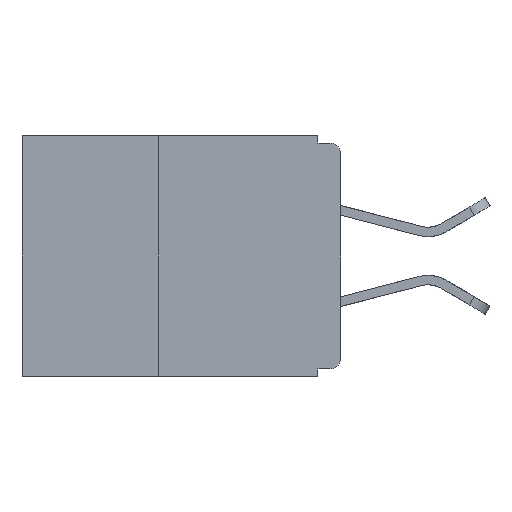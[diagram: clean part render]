
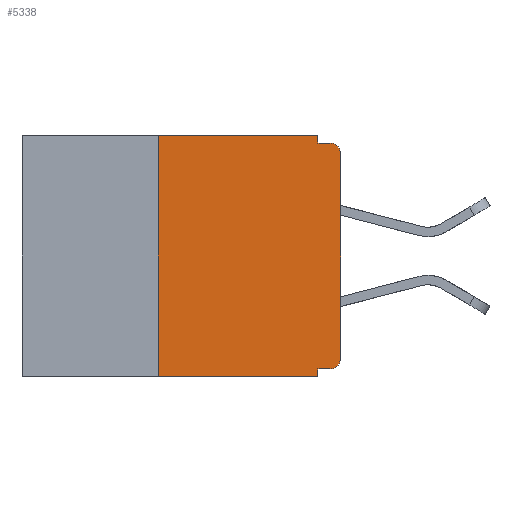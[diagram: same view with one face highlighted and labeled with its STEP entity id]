
A CAD part, left-side view. The second image highlights one B-rep face of the part: STEP entity #5338.
In plain terms, the highlighted planar face has unit normal (-1, 0, 0).
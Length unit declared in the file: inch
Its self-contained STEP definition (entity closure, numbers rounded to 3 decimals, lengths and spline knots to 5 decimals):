
#196 = VERTEX_POINT ( 'NONE', #17558 ) ;
#339 = VECTOR ( 'NONE', #9241, 39.37008 ) ;
#547 = VERTEX_POINT ( 'NONE', #24263 ) ;
#1603 = LINE ( 'NONE', #8749, #11624 ) ;
#1702 = EDGE_CURVE ( 'NONE', #196, #2056, #15099, .T. ) ;
#1730 = CARTESIAN_POINT ( 'NONE',  ( 0., 0.25, 0. ) ) ;
#2012 = CARTESIAN_POINT ( 'NONE',  ( 0., 0.25, -0.33 ) ) ;
#2056 = VERTEX_POINT ( 'NONE', #15801 ) ;
#2233 = LINE ( 'NONE', #6199, #12249 ) ;
#2402 = CIRCLE ( 'NONE', #25564, 0.015 ) ;
#2749 = ORIENTED_EDGE ( 'NONE', *, *, #4209, .T. ) ;
#2896 = CARTESIAN_POINT ( 'NONE',  ( 0., 0., -0.32 ) ) ;
#3173 = VERTEX_POINT ( 'NONE', #2012 ) ;
#3398 = LINE ( 'NONE', #2896, #12779 ) ;
#3401 = CARTESIAN_POINT ( 'NONE',  ( 0., 0.031, -0.32 ) ) ;
#3405 = ORIENTED_EDGE ( 'NONE', *, *, #19158, .F. ) ;
#4090 = EDGE_CURVE ( 'NONE', #4174, #18874, #1603, .T. ) ;
#4174 = VERTEX_POINT ( 'NONE', #6416 ) ;
#4209 = EDGE_CURVE ( 'NONE', #24738, #4174, #14375, .T. ) ;
#4511 = CARTESIAN_POINT ( 'NONE',  ( 0., 0.437, 0. ) ) ;
#4970 = ORIENTED_EDGE ( 'NONE', *, *, #14299, .T. ) ;
#4974 = VERTEX_POINT ( 'NONE', #3401 ) ;
#5245 = DIRECTION ( 'NONE',  ( 0., 0., -1. ) ) ;
#5330 = DIRECTION ( 'NONE',  ( -1., 0., 0. ) ) ;
#5338 = ADVANCED_FACE ( 'NONE', ( #14022 ), #20256, .F. ) ;
#5351 = DIRECTION ( 'NONE',  ( -1., 0., 0. ) ) ;
#5498 = CARTESIAN_POINT ( 'NONE',  ( 0., 0.015, -0.305 ) ) ;
#6107 = CARTESIAN_POINT ( 'NONE',  ( 0., 0.437, -0.33 ) ) ;
#6199 = CARTESIAN_POINT ( 'NONE',  ( 0., 0.031, -0.33 ) ) ;
#6416 = CARTESIAN_POINT ( 'NONE',  ( 0., 0., -0.305 ) ) ;
#6510 = DIRECTION ( 'NONE',  ( 1., 0., 0. ) ) ;
#6630 = AXIS2_PLACEMENT_3D ( 'NONE', #5498, #5330, #5245 ) ;
#7060 = DIRECTION ( 'NONE',  ( 0., 0., -1. ) ) ;
#7570 = LINE ( 'NONE', #6107, #25068 ) ;
#8061 = DIRECTION ( 'NONE',  ( 0., -1., 0. ) ) ;
#8165 = DIRECTION ( 'NONE',  ( 0., 0., 1. ) ) ;
#8234 = DIRECTION ( 'NONE',  ( 0., 0., -1. ) ) ;
#8249 = VECTOR ( 'NONE', #13335, 39.37008 ) ;
#8393 = ORIENTED_EDGE ( 'NONE', *, *, #1702, .F. ) ;
#8413 = ORIENTED_EDGE ( 'NONE', *, *, #14343, .F. ) ;
#8749 = CARTESIAN_POINT ( 'NONE',  ( 0., 0., 0. ) ) ;
#8942 = DIRECTION ( 'NONE',  ( 0., 1., 0. ) ) ;
#9241 = DIRECTION ( 'NONE',  ( 0., 0., 1. ) ) ;
#11624 = VECTOR ( 'NONE', #8165, 39.37008 ) ;
#12249 = VECTOR ( 'NONE', #8234, 39.37008 ) ;
#12487 = ORIENTED_EDGE ( 'NONE', *, *, #13399, .F. ) ;
#12779 = VECTOR ( 'NONE', #8942, 39.37008 ) ;
#12788 = ORIENTED_EDGE ( 'NONE', *, *, #24495, .T. ) ;
#13335 = DIRECTION ( 'NONE',  ( 0., -1., 0. ) ) ;
#13399 = EDGE_CURVE ( 'NONE', #16351, #547, #24535, .T. ) ;
#13924 = EDGE_LOOP ( 'NONE', ( #23977, #12788, #8393, #23773, #12487, #3405, #4970, #8413, #24376, #2749 ) ) ;
#14022 = FACE_OUTER_BOUND ( 'NONE', #13924, .T. ) ;
#14299 = EDGE_CURVE ( 'NONE', #3173, #17134, #7570, .T. ) ;
#14343 = EDGE_CURVE ( 'NONE', #4974, #17134, #2233, .T. ) ;
#14375 = CIRCLE ( 'NONE', #6630, 0.015 ) ;
#15099 = LINE ( 'NONE', #20082, #24827 ) ;
#15801 = CARTESIAN_POINT ( 'NONE',  ( 0., 0.015, -0.01 ) ) ;
#16240 = LINE ( 'NONE', #19032, #339 ) ;
#16351 = VERTEX_POINT ( 'NONE', #1730 ) ;
#16934 = CARTESIAN_POINT ( 'NONE',  ( 0., 0.031, 0. ) ) ;
#17134 = VERTEX_POINT ( 'NONE', #21874 ) ;
#17212 = CARTESIAN_POINT ( 'NONE',  ( 0., 0.015, -0.025 ) ) ;
#17558 = CARTESIAN_POINT ( 'NONE',  ( 0., 0.031, -0.01 ) ) ;
#18874 = VERTEX_POINT ( 'NONE', #19456 ) ;
#19032 = CARTESIAN_POINT ( 'NONE',  ( 0., 0.25, -0.33 ) ) ;
#19158 = EDGE_CURVE ( 'NONE', #3173, #16351, #16240, .T. ) ;
#19178 = DIRECTION ( 'NONE',  ( 0., 0., -1. ) ) ;
#19456 = CARTESIAN_POINT ( 'NONE',  ( 0., 0., -0.025 ) ) ;
#20082 = CARTESIAN_POINT ( 'NONE',  ( 0., 0., -0.01 ) ) ;
#20228 = DIRECTION ( 'NONE',  ( 0., -1., 0. ) ) ;
#20256 = PLANE ( 'NONE',  #21041 ) ;
#20338 = DIRECTION ( 'NONE',  ( 0., 0., -1. ) ) ;
#21041 = AXIS2_PLACEMENT_3D ( 'NONE', #4511, #6510, #20338 ) ;
#21070 = LINE ( 'NONE', #16934, #25570 ) ;
#21547 = EDGE_CURVE ( 'NONE', #24738, #4974, #3398, .T. ) ;
#21700 = CARTESIAN_POINT ( 'NONE',  ( 0., 0.015, -0.32 ) ) ;
#21874 = CARTESIAN_POINT ( 'NONE',  ( 0., 0.031, -0.33 ) ) ;
#23087 = CARTESIAN_POINT ( 'NONE',  ( 0., 0.437, 0. ) ) ;
#23260 = EDGE_CURVE ( 'NONE', #547, #196, #21070, .T. ) ;
#23773 = ORIENTED_EDGE ( 'NONE', *, *, #23260, .F. ) ;
#23977 = ORIENTED_EDGE ( 'NONE', *, *, #4090, .T. ) ;
#24263 = CARTESIAN_POINT ( 'NONE',  ( 0., 0.031, 0. ) ) ;
#24376 = ORIENTED_EDGE ( 'NONE', *, *, #21547, .F. ) ;
#24495 = EDGE_CURVE ( 'NONE', #18874, #2056, #2402, .T. ) ;
#24535 = LINE ( 'NONE', #23087, #8249 ) ;
#24738 = VERTEX_POINT ( 'NONE', #21700 ) ;
#24827 = VECTOR ( 'NONE', #20228, 39.37008 ) ;
#25068 = VECTOR ( 'NONE', #8061, 39.37008 ) ;
#25564 = AXIS2_PLACEMENT_3D ( 'NONE', #17212, #5351, #19178 ) ;
#25570 = VECTOR ( 'NONE', #7060, 39.37008 ) ;
